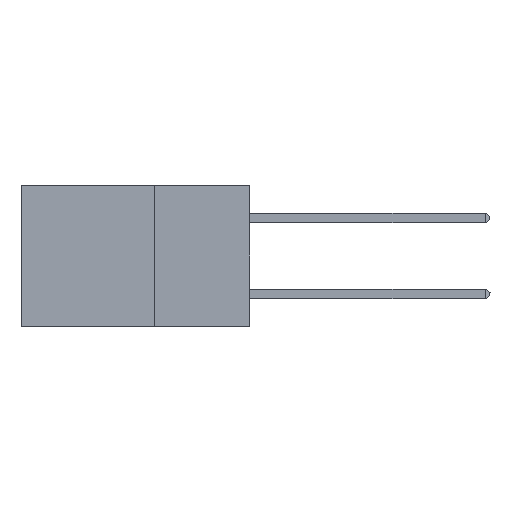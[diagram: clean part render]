
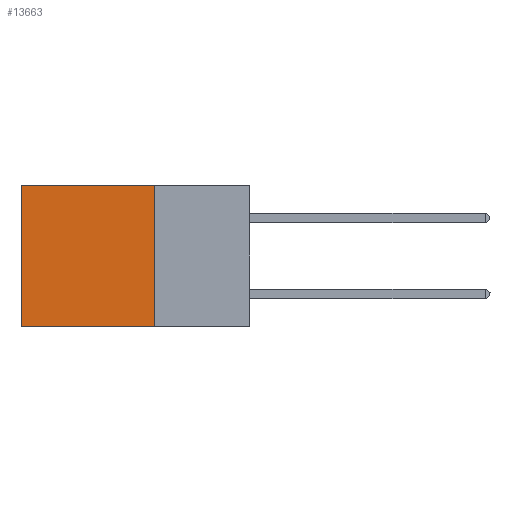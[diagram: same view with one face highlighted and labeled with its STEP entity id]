
A CAD part, left-side view. The second image highlights one B-rep face of the part: STEP entity #13663.
In plain terms, the highlighted planar face has unit normal (-1, 0, 0).
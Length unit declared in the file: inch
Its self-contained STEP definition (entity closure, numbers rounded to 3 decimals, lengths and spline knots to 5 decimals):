
#607 = CARTESIAN_POINT ( 'NONE',  ( 0.2875, 0.25, 0. ) ) ;
#704 = LINE ( 'NONE', #19662, #10144 ) ;
#817 = ORIENTED_EDGE ( 'NONE', *, *, #12537, .T. ) ;
#1404 = LINE ( 'NONE', #23625, #21480 ) ;
#3223 = DIRECTION ( 'NONE',  ( 0., 0., -1. ) ) ;
#3289 = CARTESIAN_POINT ( 'NONE',  ( 0.2875, 0.25, -0.37 ) ) ;
#5986 = DIRECTION ( 'NONE',  ( 0., 0., -1. ) ) ;
#6137 = DIRECTION ( 'NONE',  ( 1., 0., 0. ) ) ;
#6526 = CARTESIAN_POINT ( 'NONE',  ( 0.2875, 0.6, 0. ) ) ;
#7335 = EDGE_CURVE ( 'NONE', #18232, #14769, #704, .T. ) ;
#8475 = EDGE_LOOP ( 'NONE', ( #817, #21053, #16170, #24146 ) ) ;
#8798 = AXIS2_PLACEMENT_3D ( 'NONE', #22965, #6137, #5986 ) ;
#10144 = VECTOR ( 'NONE', #15776, 39.37008 ) ;
#10452 = LINE ( 'NONE', #24009, #16962 ) ;
#12528 = CARTESIAN_POINT ( 'NONE',  ( 0.2875, 0.6, 0. ) ) ;
#12537 = EDGE_CURVE ( 'NONE', #22627, #22162, #21187, .T. ) ;
#13580 = EDGE_CURVE ( 'NONE', #18232, #22627, #1404, .T. ) ;
#13663 = ADVANCED_FACE ( 'NONE', ( #19702 ), #17314, .F. ) ;
#14705 = CARTESIAN_POINT ( 'NONE',  ( 0.2875, 0.6, -0.37 ) ) ;
#14769 = VERTEX_POINT ( 'NONE', #3289 ) ;
#15776 = DIRECTION ( 'NONE',  ( 0., 0., -1. ) ) ;
#16170 = ORIENTED_EDGE ( 'NONE', *, *, #7335, .F. ) ;
#16962 = VECTOR ( 'NONE', #19982, 39.37008 ) ;
#17314 = PLANE ( 'NONE',  #8798 ) ;
#17384 = VECTOR ( 'NONE', #3223, 39.37008 ) ;
#18232 = VERTEX_POINT ( 'NONE', #607 ) ;
#19662 = CARTESIAN_POINT ( 'NONE',  ( 0.2875, 0.25, 0. ) ) ;
#19702 = FACE_OUTER_BOUND ( 'NONE', #8475, .T. ) ;
#19982 = DIRECTION ( 'NONE',  ( 0., 1., 0. ) ) ;
#21053 = ORIENTED_EDGE ( 'NONE', *, *, #24334, .F. ) ;
#21187 = LINE ( 'NONE', #6526, #17384 ) ;
#21192 = DIRECTION ( 'NONE',  ( 0., 1., 0. ) ) ;
#21480 = VECTOR ( 'NONE', #21192, 39.37008 ) ;
#22162 = VERTEX_POINT ( 'NONE', #14705 ) ;
#22627 = VERTEX_POINT ( 'NONE', #12528 ) ;
#22965 = CARTESIAN_POINT ( 'NONE',  ( 0.2875, 0.25, 0. ) ) ;
#23625 = CARTESIAN_POINT ( 'NONE',  ( 0.2875, 0.25, 0. ) ) ;
#24009 = CARTESIAN_POINT ( 'NONE',  ( 0.2875, 0.25, -0.37 ) ) ;
#24146 = ORIENTED_EDGE ( 'NONE', *, *, #13580, .T. ) ;
#24334 = EDGE_CURVE ( 'NONE', #14769, #22162, #10452, .T. ) ;
